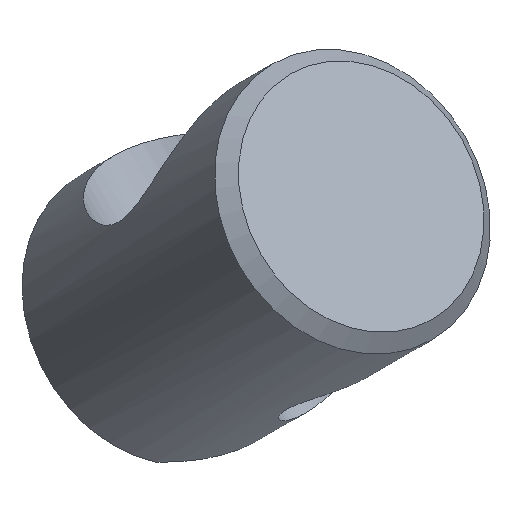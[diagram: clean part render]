
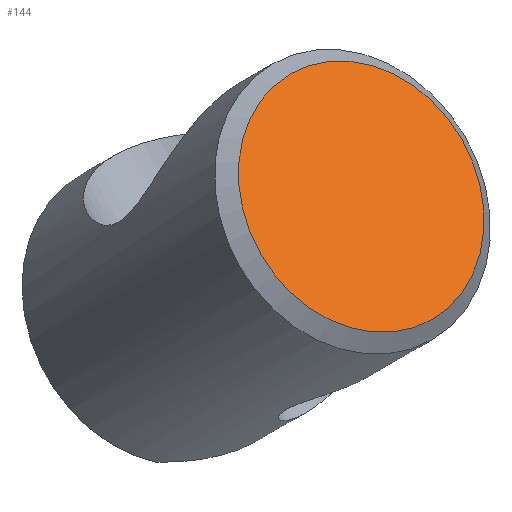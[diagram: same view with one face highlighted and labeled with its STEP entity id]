
A CAD part, isometric view. The second image highlights one B-rep face of the part: STEP entity #144.
In plain terms, the highlighted planar face has unit normal (0, -0.707, 0.707).
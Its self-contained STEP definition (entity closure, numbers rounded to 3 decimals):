
#17=PLANE('',#172);
#34=FACE_OUTER_BOUND('',#45,.T.);
#45=EDGE_LOOP('',(#116));
#63=CIRCLE('',#166,4.05);
#70=VERTEX_POINT('',#225);
#83=EDGE_CURVE('',#70,#70,#63,.T.);
#116=ORIENTED_EDGE('',*,*,#83,.F.);
#144=ADVANCED_FACE('',(#34),#17,.T.);
#166=AXIS2_PLACEMENT_3D('',#226,#186,#187);
#172=AXIS2_PLACEMENT_3D('',#322,#200,#201);
#186=DIRECTION('center_axis',(0.,0.707,-0.707));
#187=DIRECTION('ref_axis',(-1.,0.,0.));
#200=DIRECTION('center_axis',(0.,-0.707,
0.707));
#201=DIRECTION('ref_axis',(-1.,0.,0.));
#225=CARTESIAN_POINT('',(67.348,-7.022,10.703));
#226=CARTESIAN_POINT('Origin',(63.298,-7.022,10.703));
#322=CARTESIAN_POINT('Origin',(63.298,-7.022,10.703));
